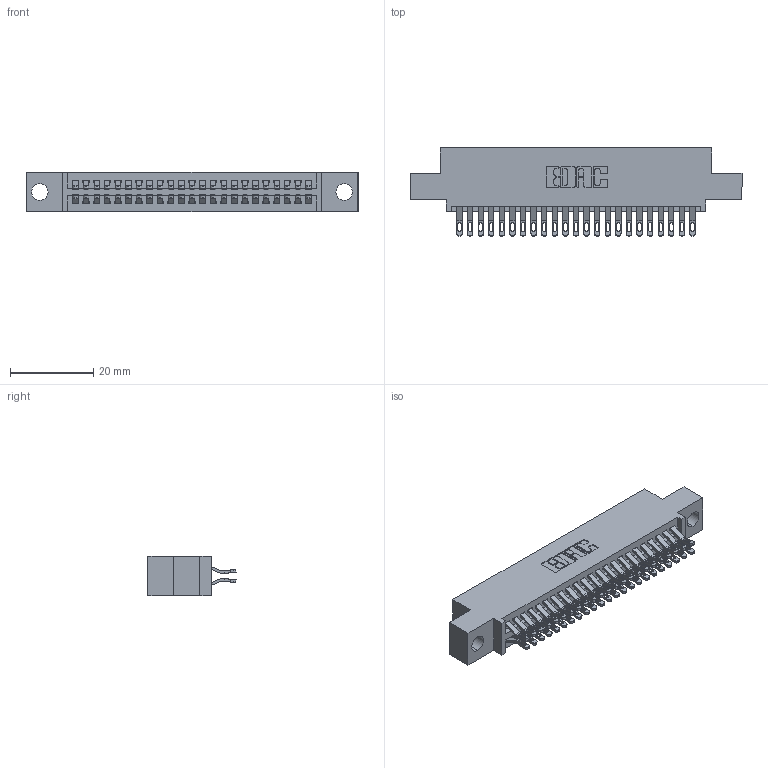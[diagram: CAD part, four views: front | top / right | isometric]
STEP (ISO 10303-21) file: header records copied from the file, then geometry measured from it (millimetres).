
FILE_DESCRIPTION (( 'STEP AP203' ), '1' );
FILE_NAME ('395-046-555-504.STEP', '2018-11-16T17:18:06', ( '' ), ( '' ), 'SwSTEP 2.0', 'SolidWorks 2016', '' );
FILE_SCHEMA (( 'CONFIG_CONTROL_DESIGN' ));
Length unit declared in the file: inch
Products named in the file (3): 395-046-555-504; 345-292-001_555 Tail; 345 Part_0.110 Offset - 0.156 Dia-TH
Assembly tree (47 placements, depth 2):
  395-046-555-504
    345 Part_0.110 Offset - 0.156 Dia-TH
    345-292-001_555 Tail  x46
Bounding box: 79.63 x 21.13 x 9.4 mm (x, y, z)
Volume: 7531.1 mm3; surface area: 11136.3 mm2
Topology: 47 solids, 47 shells, 2706 faces, 8495 edges, 5662 vertices
Faces by surface type: plane 1510, cylinder 1196
Entity records: 21065 total; most frequent: CARTESIAN_POINT 3586, ORIENTED_EDGE 3490, DIRECTION 3153, EDGE_CURVE 1745, LINE 1501, VECTOR 1501, VERTEX_POINT 1162, AXIS2_PLACEMENT_3D 826
